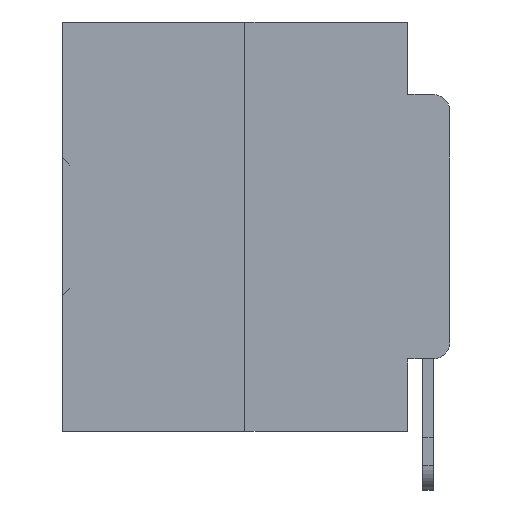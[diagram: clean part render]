
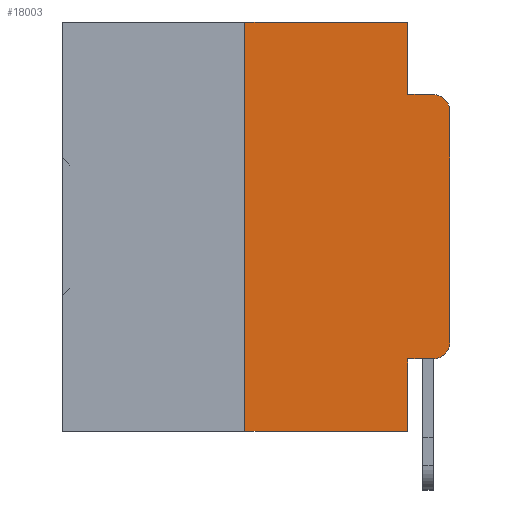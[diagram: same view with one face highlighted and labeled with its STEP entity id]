
A CAD part, left-side view. The second image highlights one B-rep face of the part: STEP entity #18003.
In plain terms, the highlighted planar face has unit normal (-1, 0, 0).
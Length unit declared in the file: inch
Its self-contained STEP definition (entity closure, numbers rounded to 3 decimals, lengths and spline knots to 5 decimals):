
#546 = CIRCLE ( 'NONE', #2283, 0.02 ) ;
#1429 = CARTESIAN_POINT ( 'NONE',  ( 0., 0., 0. ) ) ;
#1585 = DIRECTION ( 'NONE',  ( 0., 0., -1. ) ) ;
#1803 = CARTESIAN_POINT ( 'NONE',  ( 0., 0.25, 0. ) ) ;
#2283 = AXIS2_PLACEMENT_3D ( 'NONE', #36867, #20047, #2770 ) ;
#2770 = DIRECTION ( 'NONE',  ( 0., 0., -1. ) ) ;
#2881 = VERTEX_POINT ( 'NONE', #25820 ) ;
#3004 = DIRECTION ( 'NONE',  ( 0., -1., 0. ) ) ;
#3850 = VERTEX_POINT ( 'NONE', #12080 ) ;
#4709 = VERTEX_POINT ( 'NONE', #22039 ) ;
#5551 = EDGE_CURVE ( 'NONE', #2881, #4709, #546, .T. ) ;
#5785 = EDGE_CURVE ( 'NONE', #18393, #31985, #8817, .T. ) ;
#7738 = VECTOR ( 'NONE', #10982, 39.37008 ) ;
#8196 = CARTESIAN_POINT ( 'NONE',  ( 0., 0.473, -0.5 ) ) ;
#8335 = LINE ( 'NONE', #16644, #23465 ) ;
#8585 = AXIS2_PLACEMENT_3D ( 'NONE', #16896, #36540, #19737 ) ;
#8817 = CIRCLE ( 'NONE', #23467, 0.02 ) ;
#9049 = CARTESIAN_POINT ( 'NONE',  ( 0., 0.473, 0. ) ) ;
#9179 = CARTESIAN_POINT ( 'NONE',  ( 0., 0.051, -0.4115 ) ) ;
#9464 = LINE ( 'NONE', #1429, #23664 ) ;
#9467 = EDGE_CURVE ( 'NONE', #31985, #2881, #9464, .T. ) ;
#10295 = DIRECTION ( 'NONE',  ( 0., 0., 1. ) ) ;
#10537 = FACE_OUTER_BOUND ( 'NONE', #34661, .T. ) ;
#10982 = DIRECTION ( 'NONE',  ( 0., 0., -1. ) ) ;
#11167 = VERTEX_POINT ( 'NONE', #9179 ) ;
#11872 = DIRECTION ( 'NONE',  ( 0., -1., 0. ) ) ;
#12080 = CARTESIAN_POINT ( 'NONE',  ( 0., 0.051, -0.0885 ) ) ;
#13968 = DIRECTION ( 'NONE',  ( 0., -1., 0. ) ) ;
#14016 = PLANE ( 'NONE',  #8585 ) ;
#14719 = EDGE_CURVE ( 'NONE', #11167, #18393, #8335, .T. ) ;
#14745 = ORIENTED_EDGE ( 'NONE', *, *, #5785, .T. ) ;
#14813 = VECTOR ( 'NONE', #11872, 39.37008 ) ;
#15347 = CARTESIAN_POINT ( 'NONE',  ( 0., 0.02, -0.3915 ) ) ;
#16412 = DIRECTION ( 'NONE',  ( 0., 0., 1. ) ) ;
#16644 = CARTESIAN_POINT ( 'NONE',  ( 0., 0.051, -0.4115 ) ) ;
#16645 = EDGE_CURVE ( 'NONE', #11167, #32068, #31234, .T. ) ;
#16649 = VECTOR ( 'NONE', #16412, 39.37008 ) ;
#16896 = CARTESIAN_POINT ( 'NONE',  ( 0., 0.473, 0. ) ) ;
#16900 = ORIENTED_EDGE ( 'NONE', *, *, #5551, .T. ) ;
#17190 = EDGE_CURVE ( 'NONE', #30167, #32068, #33389, .T. ) ;
#17792 = ORIENTED_EDGE ( 'NONE', *, *, #27255, .F. ) ;
#18003 = ADVANCED_FACE ( 'NONE', ( #10537 ), #14016, .F. ) ;
#18197 = DIRECTION ( 'NONE',  ( 0., 0., -1. ) ) ;
#18329 = VECTOR ( 'NONE', #1585, 39.37008 ) ;
#18393 = VERTEX_POINT ( 'NONE', #24495 ) ;
#19201 = LINE ( 'NONE', #27405, #18329 ) ;
#19471 = DIRECTION ( 'NONE',  ( 0., -1., 0. ) ) ;
#19737 = DIRECTION ( 'NONE',  ( 0., 0., -1. ) ) ;
#20047 = DIRECTION ( 'NONE',  ( -1., 0., 0. ) ) ;
#20433 = ORIENTED_EDGE ( 'NONE', *, *, #22781, .F. ) ;
#20673 = CARTESIAN_POINT ( 'NONE',  ( 0., 0., -0.3915 ) ) ;
#22039 = CARTESIAN_POINT ( 'NONE',  ( 0., 0.02, -0.0885 ) ) ;
#22308 = LINE ( 'NONE', #23120, #14813 ) ;
#22590 = ORIENTED_EDGE ( 'NONE', *, *, #9467, .T. ) ;
#22781 = EDGE_CURVE ( 'NONE', #24635, #27145, #23461, .T. ) ;
#23120 = CARTESIAN_POINT ( 'NONE',  ( 0., 0.051, -0.0885 ) ) ;
#23461 = LINE ( 'NONE', #9049, #25231 ) ;
#23465 = VECTOR ( 'NONE', #19471, 39.37008 ) ;
#23467 = AXIS2_PLACEMENT_3D ( 'NONE', #15347, #35025, #18197 ) ;
#23664 = VECTOR ( 'NONE', #10295, 39.37008 ) ;
#24139 = LINE ( 'NONE', #1803, #16649 ) ;
#24382 = ORIENTED_EDGE ( 'NONE', *, *, #36643, .F. ) ;
#24495 = CARTESIAN_POINT ( 'NONE',  ( 0., 0.02, -0.4115 ) ) ;
#24635 = VERTEX_POINT ( 'NONE', #34858 ) ;
#25231 = VECTOR ( 'NONE', #3004, 39.37008 ) ;
#25820 = CARTESIAN_POINT ( 'NONE',  ( 0., 0., -0.1085 ) ) ;
#25925 = VECTOR ( 'NONE', #13968, 39.37008 ) ;
#26074 = EDGE_CURVE ( 'NONE', #30167, #24635, #24139, .T. ) ;
#27145 = VERTEX_POINT ( 'NONE', #32581 ) ;
#27255 = EDGE_CURVE ( 'NONE', #27145, #3850, #19201, .T. ) ;
#27405 = CARTESIAN_POINT ( 'NONE',  ( 0., 0.051, 0. ) ) ;
#27940 = CARTESIAN_POINT ( 'NONE',  ( 0., 0.051, 0. ) ) ;
#29312 = ORIENTED_EDGE ( 'NONE', *, *, #14719, .T. ) ;
#29655 = ORIENTED_EDGE ( 'NONE', *, *, #26074, .F. ) ;
#30167 = VERTEX_POINT ( 'NONE', #36160 ) ;
#30526 = ORIENTED_EDGE ( 'NONE', *, *, #17190, .T. ) ;
#31234 = LINE ( 'NONE', #27940, #7738 ) ;
#31985 = VERTEX_POINT ( 'NONE', #20673 ) ;
#32068 = VERTEX_POINT ( 'NONE', #35162 ) ;
#32581 = CARTESIAN_POINT ( 'NONE',  ( 0., 0.051, 0. ) ) ;
#33389 = LINE ( 'NONE', #8196, #25925 ) ;
#34575 = ORIENTED_EDGE ( 'NONE', *, *, #16645, .F. ) ;
#34661 = EDGE_LOOP ( 'NONE', ( #22590, #16900, #24382, #17792, #20433, #29655, #30526, #34575, #29312, #14745 ) ) ;
#34858 = CARTESIAN_POINT ( 'NONE',  ( 0., 0.25, 0. ) ) ;
#35025 = DIRECTION ( 'NONE',  ( -1., 0., 0. ) ) ;
#35162 = CARTESIAN_POINT ( 'NONE',  ( 0., 0.051, -0.5 ) ) ;
#36160 = CARTESIAN_POINT ( 'NONE',  ( 0., 0.25, -0.5 ) ) ;
#36540 = DIRECTION ( 'NONE',  ( 1., 0., 0. ) ) ;
#36643 = EDGE_CURVE ( 'NONE', #3850, #4709, #22308, .T. ) ;
#36867 = CARTESIAN_POINT ( 'NONE',  ( 0., 0.02, -0.1085 ) ) ;
